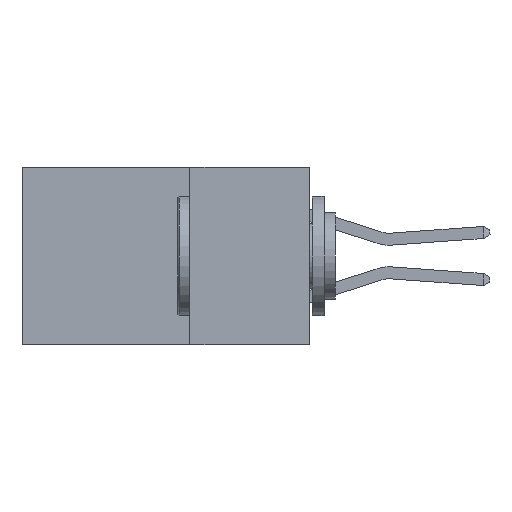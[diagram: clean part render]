
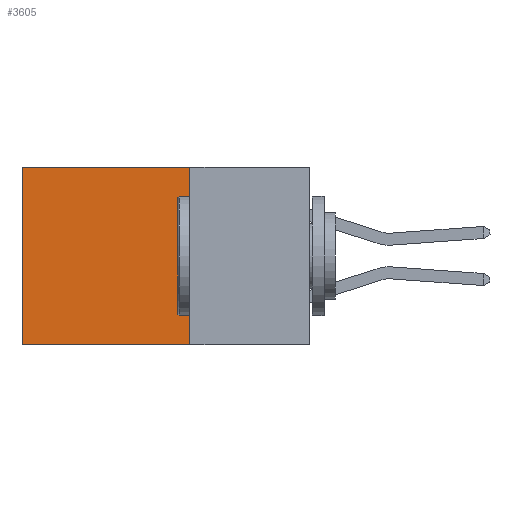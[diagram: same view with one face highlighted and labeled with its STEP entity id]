
A CAD part, left-side view. The second image highlights one B-rep face of the part: STEP entity #3605.
In plain terms, the highlighted planar face has unit normal (-1, 0, 0).
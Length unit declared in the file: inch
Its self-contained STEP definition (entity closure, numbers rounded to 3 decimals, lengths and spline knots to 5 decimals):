
#36 = AXIS2_PLACEMENT_3D ( 'NONE', #16382, #12202, #6010 ) ;
#1944 = LINE ( 'NONE', #26224, #4584 ) ;
#2363 = DIRECTION ( 'NONE',  ( 0., 1., 0. ) ) ;
#3082 = EDGE_CURVE ( 'NONE', #14228, #24517, #12438, .T. ) ;
#3605 = ADVANCED_FACE ( 'NONE', ( #23746 ), #12857, .F. ) ;
#4112 = EDGE_CURVE ( 'NONE', #15524, #14228, #1944, .T. ) ;
#4333 = EDGE_CURVE ( 'NONE', #15524, #13063, #19510, .T. ) ;
#4584 = VECTOR ( 'NONE', #5576, 39.37008 ) ;
#4875 = ORIENTED_EDGE ( 'NONE', *, *, #4112, .F. ) ;
#5576 = DIRECTION ( 'NONE',  ( 0., 0., -1. ) ) ;
#6010 = DIRECTION ( 'NONE',  ( 0., 0., -1. ) ) ;
#6922 = EDGE_LOOP ( 'NONE', ( #20462, #9602, #4875, #26279 ) ) ;
#9602 = ORIENTED_EDGE ( 'NONE', *, *, #3082, .F. ) ;
#10190 = CARTESIAN_POINT ( 'NONE',  ( 0.298, 0.25, -0.37 ) ) ;
#12202 = DIRECTION ( 'NONE',  ( 1., 0., 0. ) ) ;
#12438 = LINE ( 'NONE', #12936, #15710 ) ;
#12531 = CARTESIAN_POINT ( 'NONE',  ( 0.298, 0.6, 0. ) ) ;
#12857 = PLANE ( 'NONE',  #36 ) ;
#12936 = CARTESIAN_POINT ( 'NONE',  ( 0.298, 0.25, -0.37 ) ) ;
#13063 = VERTEX_POINT ( 'NONE', #13840 ) ;
#13840 = CARTESIAN_POINT ( 'NONE',  ( 0.298, 0.6, 0. ) ) ;
#14228 = VERTEX_POINT ( 'NONE', #10190 ) ;
#15030 = DIRECTION ( 'NONE',  ( 0., 1., 0. ) ) ;
#15524 = VERTEX_POINT ( 'NONE', #25402 ) ;
#15710 = VECTOR ( 'NONE', #15030, 39.37008 ) ;
#16382 = CARTESIAN_POINT ( 'NONE',  ( 0.298, 0.25, 0. ) ) ;
#16880 = DIRECTION ( 'NONE',  ( 0., 0., -1. ) ) ;
#16914 = EDGE_CURVE ( 'NONE', #13063, #24517, #22933, .T. ) ;
#18888 = CARTESIAN_POINT ( 'NONE',  ( 0.298, 0.6, -0.37 ) ) ;
#19510 = LINE ( 'NONE', #23271, #25332 ) ;
#20462 = ORIENTED_EDGE ( 'NONE', *, *, #16914, .T. ) ;
#22933 = LINE ( 'NONE', #12531, #24855 ) ;
#23271 = CARTESIAN_POINT ( 'NONE',  ( 0.298, 0.25, 0. ) ) ;
#23746 = FACE_OUTER_BOUND ( 'NONE', #6922, .T. ) ;
#24517 = VERTEX_POINT ( 'NONE', #18888 ) ;
#24855 = VECTOR ( 'NONE', #16880, 39.37008 ) ;
#25332 = VECTOR ( 'NONE', #2363, 39.37008 ) ;
#25402 = CARTESIAN_POINT ( 'NONE',  ( 0.298, 0.25, 0. ) ) ;
#26224 = CARTESIAN_POINT ( 'NONE',  ( 0.298, 0.25, 0. ) ) ;
#26279 = ORIENTED_EDGE ( 'NONE', *, *, #4333, .T. ) ;
